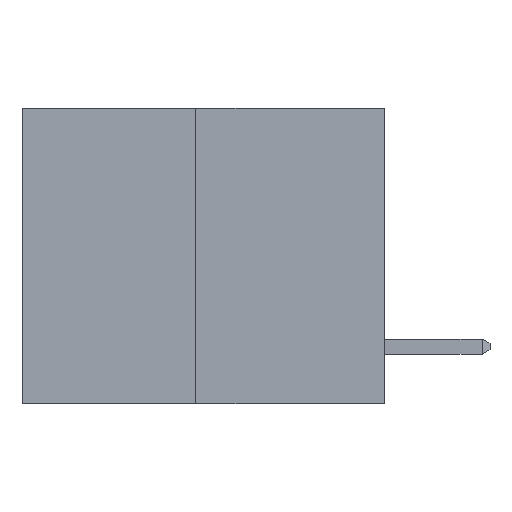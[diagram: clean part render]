
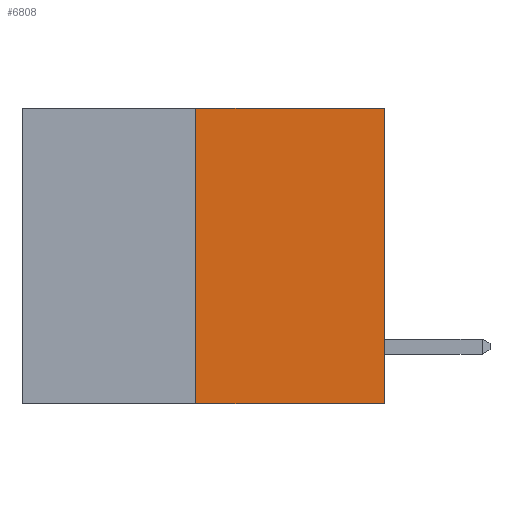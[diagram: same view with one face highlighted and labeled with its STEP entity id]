
A CAD part, left-side view. The second image highlights one B-rep face of the part: STEP entity #6808.
In plain terms, the highlighted planar face has unit normal (-1, 0, 0).
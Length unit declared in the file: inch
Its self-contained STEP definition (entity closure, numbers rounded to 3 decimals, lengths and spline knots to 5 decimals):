
#280 = VECTOR ( 'NONE', #1924, 39.37008 ) ;
#286 = ORIENTED_EDGE ( 'NONE', *, *, #3469, .T. ) ;
#429 = DIRECTION ( 'NONE',  ( 0., 0., 1. ) ) ;
#465 = CARTESIAN_POINT ( 'NONE',  ( 0., 0.312, -0.49 ) ) ;
#578 = CARTESIAN_POINT ( 'NONE',  ( 0., 0.6, 0. ) ) ;
#580 = CARTESIAN_POINT ( 'NONE',  ( 0., 0., -0.49 ) ) ;
#1331 = AXIS2_PLACEMENT_3D ( 'NONE', #5980, #8117, #3300 ) ;
#1423 = EDGE_CURVE ( 'NONE', #4254, #4228, #1561, .T. ) ;
#1561 = LINE ( 'NONE', #1727, #1662 ) ;
#1601 = EDGE_CURVE ( 'NONE', #5528, #2859, #7722, .T. ) ;
#1662 = VECTOR ( 'NONE', #8151, 39.37008 ) ;
#1688 = LINE ( 'NONE', #578, #280 ) ;
#1727 = CARTESIAN_POINT ( 'NONE',  ( 0., 0., 0. ) ) ;
#1732 = ORIENTED_EDGE ( 'NONE', *, *, #7835, .F. ) ;
#1884 = VECTOR ( 'NONE', #7496, 39.37008 ) ;
#1918 = CARTESIAN_POINT ( 'NONE',  ( 0., 0.312, 0. ) ) ;
#1924 = DIRECTION ( 'NONE',  ( 0., -1., 0. ) ) ;
#2418 = ORIENTED_EDGE ( 'NONE', *, *, #1423, .T. ) ;
#2725 = FACE_OUTER_BOUND ( 'NONE', #6694, .T. ) ;
#2776 = LINE ( 'NONE', #4058, #1884 ) ;
#2859 = VERTEX_POINT ( 'NONE', #1918 ) ;
#3300 = DIRECTION ( 'NONE',  ( 0., 0., -1. ) ) ;
#3469 = EDGE_CURVE ( 'NONE', #5528, #4254, #2776, .T. ) ;
#4058 = CARTESIAN_POINT ( 'NONE',  ( 0., 0.6, -0.49 ) ) ;
#4228 = VERTEX_POINT ( 'NONE', #5361 ) ;
#4254 = VERTEX_POINT ( 'NONE', #580 ) ;
#5361 = CARTESIAN_POINT ( 'NONE',  ( 0., 0., 0. ) ) ;
#5528 = VERTEX_POINT ( 'NONE', #6567 ) ;
#5980 = CARTESIAN_POINT ( 'NONE',  ( 0., 0.6, 0. ) ) ;
#6544 = PLANE ( 'NONE',  #1331 ) ;
#6567 = CARTESIAN_POINT ( 'NONE',  ( 0., 0.312, -0.49 ) ) ;
#6694 = EDGE_LOOP ( 'NONE', ( #8734, #286, #2418, #1732 ) ) ;
#6808 = ADVANCED_FACE ( 'NONE', ( #2725 ), #6544, .F. ) ;
#7496 = DIRECTION ( 'NONE',  ( 0., -1., 0. ) ) ;
#7722 = LINE ( 'NONE', #465, #8032 ) ;
#7835 = EDGE_CURVE ( 'NONE', #2859, #4228, #1688, .T. ) ;
#8032 = VECTOR ( 'NONE', #429, 39.37008 ) ;
#8117 = DIRECTION ( 'NONE',  ( 1., 0., 0. ) ) ;
#8151 = DIRECTION ( 'NONE',  ( 0., 0., 1. ) ) ;
#8734 = ORIENTED_EDGE ( 'NONE', *, *, #1601, .F. ) ;
